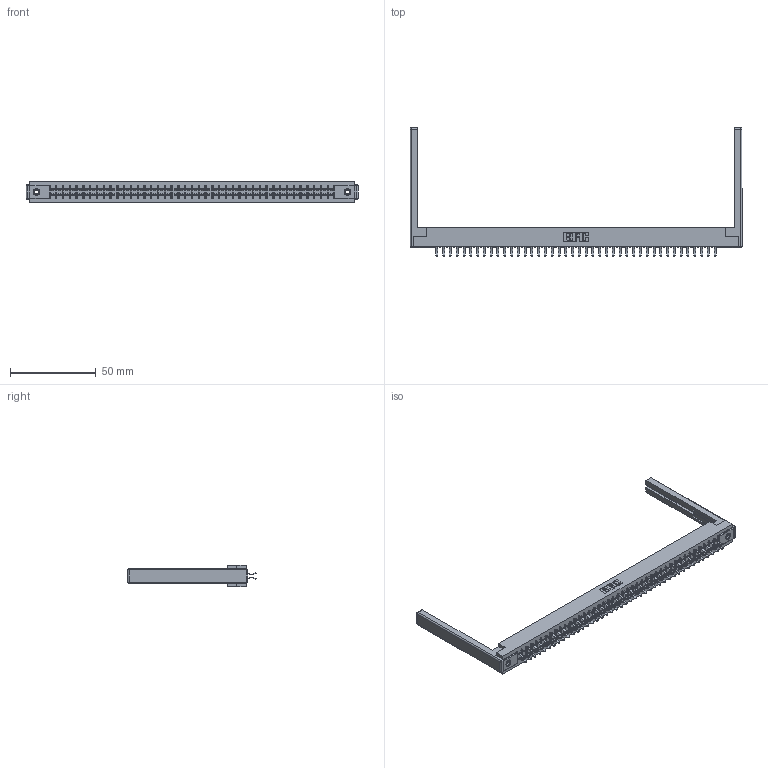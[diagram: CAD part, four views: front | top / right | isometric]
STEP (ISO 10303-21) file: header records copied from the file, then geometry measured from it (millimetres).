
FILE_DESCRIPTION (( 'STEP AP203' ), '1' );
FILE_NAME ('355-084-556-568.STEP', '2019-09-13T16:21:48', ( '' ), ( '' ), 'SwSTEP 2.0', 'SolidWorks 2016', '' );
FILE_SCHEMA (( 'CONFIG_CONTROL_DESIGN' ));
Length unit declared in the file: inch
Products named in the file (5): 307-220-068; 345-250-001_345-250-001-102; 305-290-001_556; 355-084-556-568; 305 Part_.156 Dia
Assembly tree (89 placements, depth 2):
  355-084-556-568
    305 Part_.156 Dia
    305-290-001_556  x84
    345-250-001_345-250-001-102  x2
    307-220-068  x2
Bounding box: 193.85 x 74.93 x 12.7 mm (x, y, z)
Volume: 24020.1 mm3; surface area: 29901.3 mm2
Topology: 89 solids, 89 shells, 4974 faces, 14272 edges, 9268 vertices
Faces by surface type: plane 2760, cylinder 2022, sphere 176, cone 12, torus 4
Entity records: 48456 total; most frequent: CARTESIAN_POINT 7993, ORIENTED_EDGE 7926, DIRECTION 7755, EDGE_CURVE 3963, VECTOR 3191, LINE 3191, VERTEX_POINT 2520, AXIS2_PLACEMENT_3D 2282
